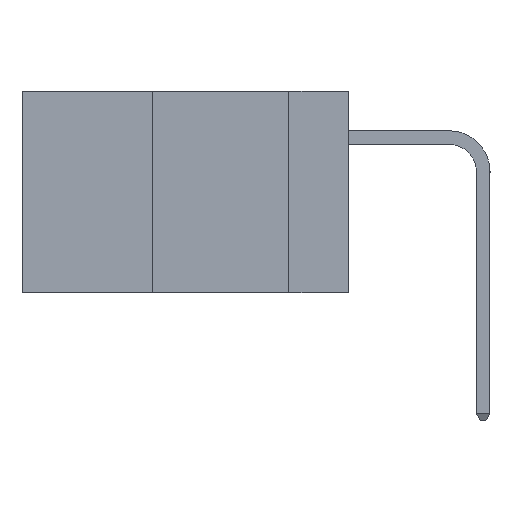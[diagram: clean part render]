
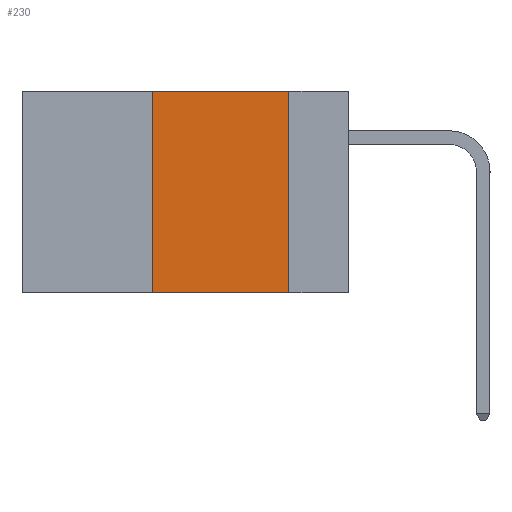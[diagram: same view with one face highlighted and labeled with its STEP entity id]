
A CAD part, left-side view. The second image highlights one B-rep face of the part: STEP entity #230.
In plain terms, the highlighted planar face has unit normal (-1, 0, 0).
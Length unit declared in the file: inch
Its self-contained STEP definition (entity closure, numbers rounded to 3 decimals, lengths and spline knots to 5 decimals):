
#230 = ADVANCED_FACE ( 'NONE', ( #8625 ), #764, .F. ) ;
#241 = DIRECTION ( 'NONE',  ( 0., 0., 1. ) ) ;
#400 = AXIS2_PLACEMENT_3D ( 'NONE', #12020, #1934, #2279 ) ;
#764 = PLANE ( 'NONE',  #400 ) ;
#855 = VECTOR ( 'NONE', #1812, 39.37008 ) ;
#905 = CARTESIAN_POINT ( 'NONE',  ( 0., 0.11, 0. ) ) ;
#1749 = DIRECTION ( 'NONE',  ( 0., -1., 0. ) ) ;
#1812 = DIRECTION ( 'NONE',  ( 0., -1., 0. ) ) ;
#1934 = DIRECTION ( 'NONE',  ( 1., 0., 0. ) ) ;
#2279 = DIRECTION ( 'NONE',  ( 0., 0., -1. ) ) ;
#2543 = VECTOR ( 'NONE', #241, 39.37008 ) ;
#2611 = VERTEX_POINT ( 'NONE', #905 ) ;
#3379 = EDGE_LOOP ( 'NONE', ( #11796, #7014, #9820, #7608 ) ) ;
#3560 = CARTESIAN_POINT ( 'NONE',  ( 0., 0.11, 0. ) ) ;
#4774 = VERTEX_POINT ( 'NONE', #12288 ) ;
#5135 = VECTOR ( 'NONE', #11207, 39.37008 ) ;
#5935 = EDGE_CURVE ( 'NONE', #4774, #9278, #9917, .T. ) ;
#6562 = CARTESIAN_POINT ( 'NONE',  ( 0., 0.6, -0.37 ) ) ;
#7014 = ORIENTED_EDGE ( 'NONE', *, *, #10973, .F. ) ;
#7126 = EDGE_CURVE ( 'NONE', #2611, #9278, #7673, .T. ) ;
#7134 = CARTESIAN_POINT ( 'NONE',  ( 0., 0.36, 0. ) ) ;
#7603 = CARTESIAN_POINT ( 'NONE',  ( 0., 0.36, 0. ) ) ;
#7604 = EDGE_CURVE ( 'NONE', #4774, #12172, #9872, .T. ) ;
#7608 = ORIENTED_EDGE ( 'NONE', *, *, #5935, .T. ) ;
#7673 = LINE ( 'NONE', #3560, #5135 ) ;
#8625 = FACE_OUTER_BOUND ( 'NONE', #3379, .T. ) ;
#9030 = CARTESIAN_POINT ( 'NONE',  ( 0., 0.11, -0.37 ) ) ;
#9278 = VERTEX_POINT ( 'NONE', #9030 ) ;
#9521 = CARTESIAN_POINT ( 'NONE',  ( 0., 0.6, 0. ) ) ;
#9820 = ORIENTED_EDGE ( 'NONE', *, *, #7604, .F. ) ;
#9872 = LINE ( 'NONE', #7134, #2543 ) ;
#9917 = LINE ( 'NONE', #6562, #12198 ) ;
#10973 = EDGE_CURVE ( 'NONE', #12172, #2611, #11783, .T. ) ;
#11207 = DIRECTION ( 'NONE',  ( 0., 0., -1. ) ) ;
#11783 = LINE ( 'NONE', #9521, #855 ) ;
#11796 = ORIENTED_EDGE ( 'NONE', *, *, #7126, .F. ) ;
#12020 = CARTESIAN_POINT ( 'NONE',  ( 0., 0.6, 0. ) ) ;
#12172 = VERTEX_POINT ( 'NONE', #7603 ) ;
#12198 = VECTOR ( 'NONE', #1749, 39.37008 ) ;
#12288 = CARTESIAN_POINT ( 'NONE',  ( 0., 0.36, -0.37 ) ) ;
